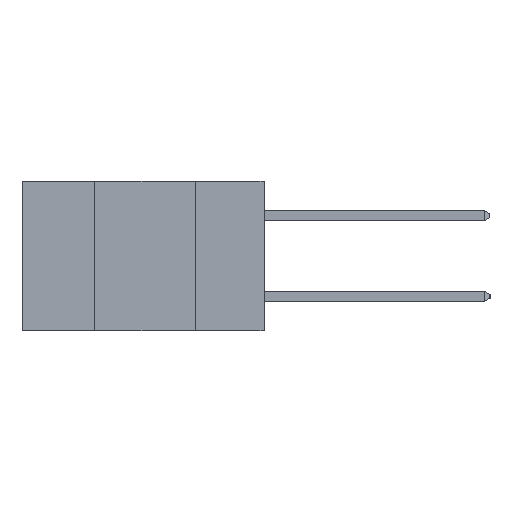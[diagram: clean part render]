
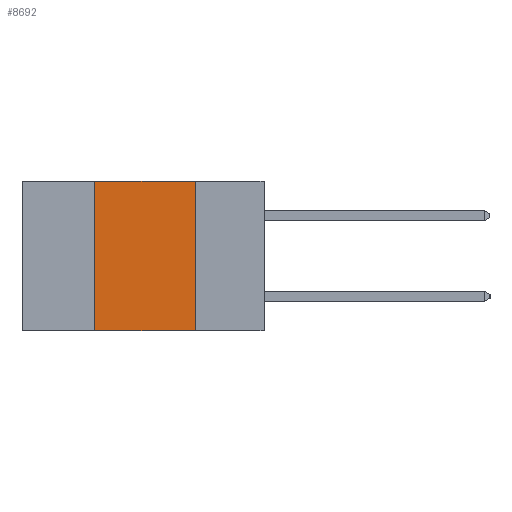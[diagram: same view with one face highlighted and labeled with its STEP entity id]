
A CAD part, left-side view. The second image highlights one B-rep face of the part: STEP entity #8692.
In plain terms, the highlighted planar face has unit normal (-1, 0, 0).
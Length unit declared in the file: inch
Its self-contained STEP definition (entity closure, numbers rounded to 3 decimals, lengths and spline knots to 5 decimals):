
#66 = ORIENTED_EDGE ( 'NONE', *, *, #6213, .T. ) ;
#333 = ORIENTED_EDGE ( 'NONE', *, *, #4229, .F. ) ;
#456 = LINE ( 'NONE', #7893, #7013 ) ;
#596 = CARTESIAN_POINT ( 'NONE',  ( 0., 0.42, 0. ) ) ;
#908 = VECTOR ( 'NONE', #1408, 39.37008 ) ;
#1125 = DIRECTION ( 'NONE',  ( 0., -1., 0. ) ) ;
#1380 = AXIS2_PLACEMENT_3D ( 'NONE', #1931, #10278, #5350 ) ;
#1408 = DIRECTION ( 'NONE',  ( 0., 0., -1. ) ) ;
#1580 = CARTESIAN_POINT ( 'NONE',  ( 0., 0.17, -0.37 ) ) ;
#1931 = CARTESIAN_POINT ( 'NONE',  ( 0., 0.6, 0. ) ) ;
#2004 = ORIENTED_EDGE ( 'NONE', *, *, #3267, .F. ) ;
#2288 = VECTOR ( 'NONE', #7964, 39.37008 ) ;
#2419 = CARTESIAN_POINT ( 'NONE',  ( 0., 0.42, -0.37 ) ) ;
#2670 = EDGE_LOOP ( 'NONE', ( #333, #4652, #2004, #66 ) ) ;
#3185 = LINE ( 'NONE', #1580, #908 ) ;
#3267 = EDGE_CURVE ( 'NONE', #10650, #8442, #6836, .T. ) ;
#4229 = EDGE_CURVE ( 'NONE', #4470, #5000, #3185, .T. ) ;
#4470 = VERTEX_POINT ( 'NONE', #7720 ) ;
#4484 = PLANE ( 'NONE',  #1380 ) ;
#4652 = ORIENTED_EDGE ( 'NONE', *, *, #5928, .F. ) ;
#4969 = CARTESIAN_POINT ( 'NONE',  ( 0., 0.17, -0.37 ) ) ;
#5000 = VERTEX_POINT ( 'NONE', #4969 ) ;
#5350 = DIRECTION ( 'NONE',  ( 0., 0., -1. ) ) ;
#5928 = EDGE_CURVE ( 'NONE', #8442, #4470, #456, .T. ) ;
#6213 = EDGE_CURVE ( 'NONE', #10650, #5000, #6624, .T. ) ;
#6624 = LINE ( 'NONE', #8211, #10693 ) ;
#6836 = LINE ( 'NONE', #7902, #2288 ) ;
#7013 = VECTOR ( 'NONE', #1125, 39.37008 ) ;
#7595 = FACE_OUTER_BOUND ( 'NONE', #2670, .T. ) ;
#7720 = CARTESIAN_POINT ( 'NONE',  ( 0., 0.17, 0. ) ) ;
#7893 = CARTESIAN_POINT ( 'NONE',  ( 0., 0.6, 0. ) ) ;
#7902 = CARTESIAN_POINT ( 'NONE',  ( 0., 0.42, -0.37 ) ) ;
#7964 = DIRECTION ( 'NONE',  ( 0., 0., 1. ) ) ;
#8211 = CARTESIAN_POINT ( 'NONE',  ( 0., 0.6, -0.37 ) ) ;
#8442 = VERTEX_POINT ( 'NONE', #596 ) ;
#8692 = ADVANCED_FACE ( 'NONE', ( #7595 ), #4484, .F. ) ;
#10278 = DIRECTION ( 'NONE',  ( 1., 0., 0. ) ) ;
#10650 = VERTEX_POINT ( 'NONE', #2419 ) ;
#10669 = DIRECTION ( 'NONE',  ( 0., -1., 0. ) ) ;
#10693 = VECTOR ( 'NONE', #10669, 39.37008 ) ;
